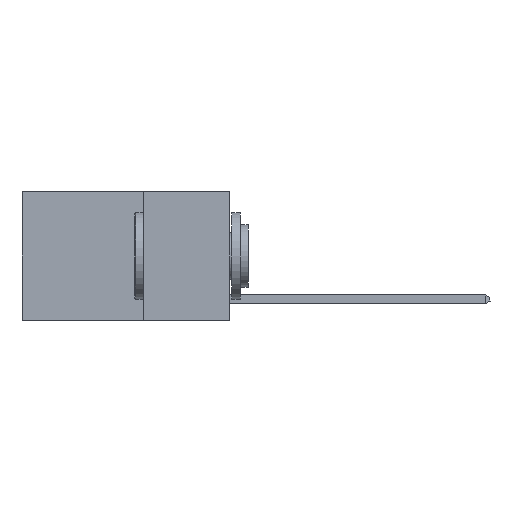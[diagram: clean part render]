
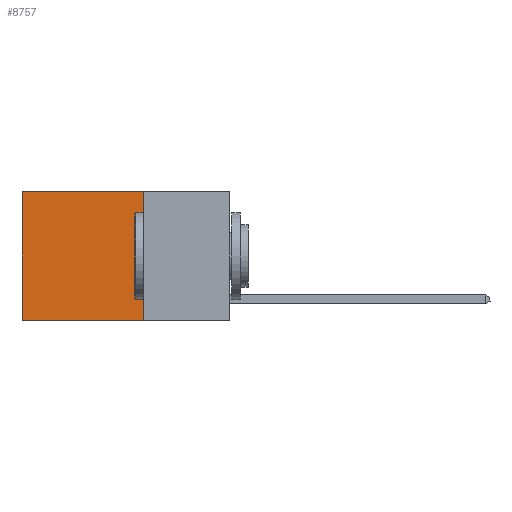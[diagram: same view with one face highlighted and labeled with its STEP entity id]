
A CAD part, left-side view. The second image highlights one B-rep face of the part: STEP entity #8757.
In plain terms, the highlighted planar face has unit normal (-1, 0, 0).
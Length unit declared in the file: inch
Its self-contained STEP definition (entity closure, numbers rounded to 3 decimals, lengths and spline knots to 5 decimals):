
#347 = VECTOR ( 'NONE', #8773, 39.37008 ) ;
#883 = AXIS2_PLACEMENT_3D ( 'NONE', #2630, #11653, #4891 ) ;
#916 = EDGE_CURVE ( 'NONE', #5241, #10326, #10751, .T. ) ;
#1556 = CARTESIAN_POINT ( 'NONE',  ( 0.2625, 0.25, 0. ) ) ;
#2335 = CARTESIAN_POINT ( 'NONE',  ( 0.2625, 0.25, -0.37 ) ) ;
#2561 = ORIENTED_EDGE ( 'NONE', *, *, #5507, .F. ) ;
#2630 = CARTESIAN_POINT ( 'NONE',  ( 0.2625, 0.25, 0. ) ) ;
#3415 = VECTOR ( 'NONE', #8315, 39.37008 ) ;
#3441 = LINE ( 'NONE', #4271, #347 ) ;
#3461 = VERTEX_POINT ( 'NONE', #5311 ) ;
#3769 = PLANE ( 'NONE',  #883 ) ;
#4152 = VERTEX_POINT ( 'NONE', #2335 ) ;
#4271 = CARTESIAN_POINT ( 'NONE',  ( 0.2625, 0.25, -0.37 ) ) ;
#4760 = VECTOR ( 'NONE', #9465, 39.37008 ) ;
#4891 = DIRECTION ( 'NONE',  ( 0., 0., -1. ) ) ;
#5068 = ORIENTED_EDGE ( 'NONE', *, *, #14527, .F. ) ;
#5241 = VERTEX_POINT ( 'NONE', #9470 ) ;
#5311 = CARTESIAN_POINT ( 'NONE',  ( 0.2625, 0.25, 0. ) ) ;
#5507 = EDGE_CURVE ( 'NONE', #4152, #10326, #3441, .T. ) ;
#6331 = CARTESIAN_POINT ( 'NONE',  ( 0.2625, 0.6, -0.37 ) ) ;
#6925 = ORIENTED_EDGE ( 'NONE', *, *, #916, .T. ) ;
#7327 = FACE_OUTER_BOUND ( 'NONE', #7962, .T. ) ;
#7962 = EDGE_LOOP ( 'NONE', ( #6925, #2561, #5068, #8175 ) ) ;
#8175 = ORIENTED_EDGE ( 'NONE', *, *, #9168, .T. ) ;
#8315 = DIRECTION ( 'NONE',  ( 0., 0., -1. ) ) ;
#8757 = ADVANCED_FACE ( 'NONE', ( #7327 ), #3769, .F. ) ;
#8773 = DIRECTION ( 'NONE',  ( 0., 1., 0. ) ) ;
#8944 = CARTESIAN_POINT ( 'NONE',  ( 0.2625, 0.25, 0. ) ) ;
#9168 = EDGE_CURVE ( 'NONE', #3461, #5241, #13960, .T. ) ;
#9465 = DIRECTION ( 'NONE',  ( 0., 0., -1. ) ) ;
#9470 = CARTESIAN_POINT ( 'NONE',  ( 0.2625, 0.6, 0. ) ) ;
#9613 = CARTESIAN_POINT ( 'NONE',  ( 0.2625, 0.6, 0. ) ) ;
#10326 = VERTEX_POINT ( 'NONE', #6331 ) ;
#10751 = LINE ( 'NONE', #9613, #4760 ) ;
#11042 = VECTOR ( 'NONE', #12329, 39.37008 ) ;
#11653 = DIRECTION ( 'NONE',  ( 1., 0., 0. ) ) ;
#12329 = DIRECTION ( 'NONE',  ( 0., 1., 0. ) ) ;
#12417 = LINE ( 'NONE', #1556, #3415 ) ;
#13960 = LINE ( 'NONE', #8944, #11042 ) ;
#14527 = EDGE_CURVE ( 'NONE', #3461, #4152, #12417, .T. ) ;
